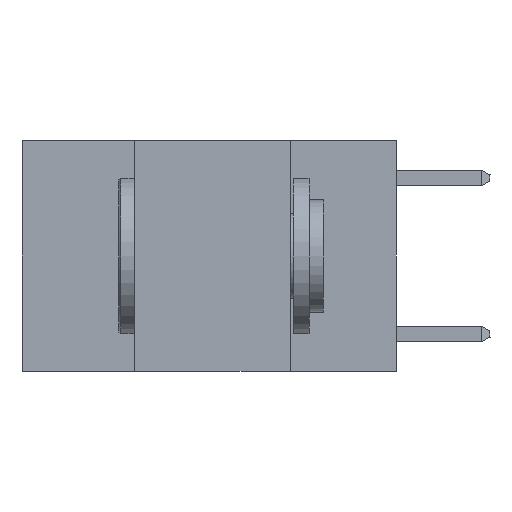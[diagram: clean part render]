
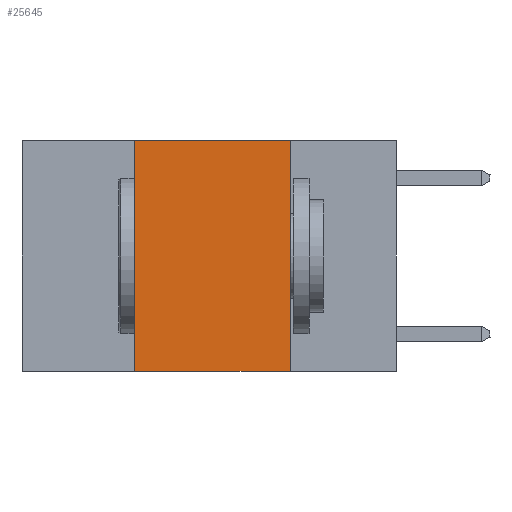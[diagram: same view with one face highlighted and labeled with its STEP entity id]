
A CAD part, left-side view. The second image highlights one B-rep face of the part: STEP entity #25645.
In plain terms, the highlighted planar face has unit normal (-1, 0, 0).
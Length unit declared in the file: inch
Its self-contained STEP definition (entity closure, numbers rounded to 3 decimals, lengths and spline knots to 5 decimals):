
#248 = DIRECTION ( 'NONE',  ( 0., 0., -1. ) ) ;
#1782 = VECTOR ( 'NONE', #7063, 39.37008 ) ;
#3880 = DIRECTION ( 'NONE',  ( 0., -1., 0. ) ) ;
#4482 = ORIENTED_EDGE ( 'NONE', *, *, #18811, .T. ) ;
#4709 = CARTESIAN_POINT ( 'NONE',  ( 0., 0.17, 0. ) ) ;
#5191 = CARTESIAN_POINT ( 'NONE',  ( 0., 0.42, 0. ) ) ;
#7063 = DIRECTION ( 'NONE',  ( 0., -1., 0. ) ) ;
#7172 = EDGE_LOOP ( 'NONE', ( #10089, #20490, #25997, #4482 ) ) ;
#7906 = CARTESIAN_POINT ( 'NONE',  ( 0., 0.6, -0.37 ) ) ;
#7915 = LINE ( 'NONE', #19779, #22593 ) ;
#8097 = EDGE_CURVE ( 'NONE', #11789, #22456, #19961, .T. ) ;
#10089 = ORIENTED_EDGE ( 'NONE', *, *, #10441, .F. ) ;
#10262 = LINE ( 'NONE', #12479, #24154 ) ;
#10441 = EDGE_CURVE ( 'NONE', #22456, #18701, #7915, .T. ) ;
#11542 = VECTOR ( 'NONE', #3880, 39.37008 ) ;
#11789 = VERTEX_POINT ( 'NONE', #5191 ) ;
#11799 = CARTESIAN_POINT ( 'NONE',  ( 0., 0.6, 0. ) ) ;
#12462 = FACE_OUTER_BOUND ( 'NONE', #7172, .T. ) ;
#12479 = CARTESIAN_POINT ( 'NONE',  ( 0., 0.42, 0. ) ) ;
#16151 = CARTESIAN_POINT ( 'NONE',  ( 0., 0.42, -0.37 ) ) ;
#17078 = CARTESIAN_POINT ( 'NONE',  ( 0., 0.6, 0. ) ) ;
#18289 = DIRECTION ( 'NONE',  ( 0., 0., 1. ) ) ;
#18701 = VERTEX_POINT ( 'NONE', #25592 ) ;
#18811 = EDGE_CURVE ( 'NONE', #19379, #18701, #19884, .T. ) ;
#18932 = DIRECTION ( 'NONE',  ( 1., 0., 0. ) ) ;
#19379 = VERTEX_POINT ( 'NONE', #16151 ) ;
#19779 = CARTESIAN_POINT ( 'NONE',  ( 0., 0.17, 0. ) ) ;
#19884 = LINE ( 'NONE', #7906, #1782 ) ;
#19961 = LINE ( 'NONE', #11799, #11542 ) ;
#20490 = ORIENTED_EDGE ( 'NONE', *, *, #8097, .F. ) ;
#20503 = PLANE ( 'NONE',  #21695 ) ;
#20641 = DIRECTION ( 'NONE',  ( 0., 0., -1. ) ) ;
#21695 = AXIS2_PLACEMENT_3D ( 'NONE', #17078, #18932, #20641 ) ;
#22368 = EDGE_CURVE ( 'NONE', #19379, #11789, #10262, .T. ) ;
#22456 = VERTEX_POINT ( 'NONE', #4709 ) ;
#22593 = VECTOR ( 'NONE', #248, 39.37008 ) ;
#24154 = VECTOR ( 'NONE', #18289, 39.37008 ) ;
#25592 = CARTESIAN_POINT ( 'NONE',  ( 0., 0.17, -0.37 ) ) ;
#25645 = ADVANCED_FACE ( 'NONE', ( #12462 ), #20503, .F. ) ;
#25997 = ORIENTED_EDGE ( 'NONE', *, *, #22368, .F. ) ;
